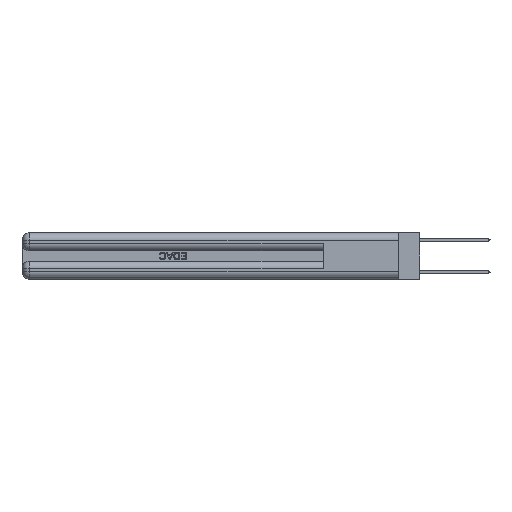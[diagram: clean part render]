
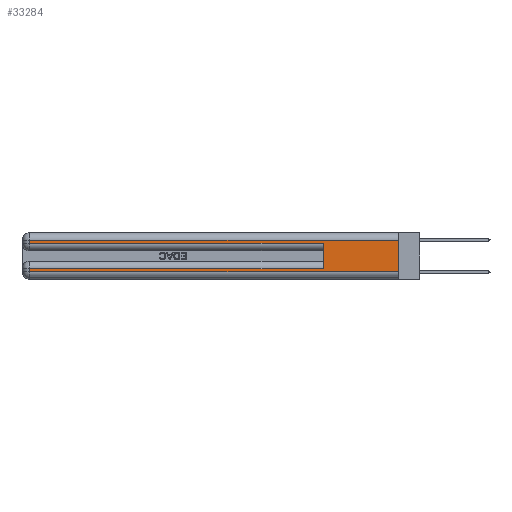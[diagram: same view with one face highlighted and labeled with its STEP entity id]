
A CAD part, left-side view. The second image highlights one B-rep face of the part: STEP entity #33284.
In plain terms, the highlighted planar face has unit normal (-1, 0, 0).
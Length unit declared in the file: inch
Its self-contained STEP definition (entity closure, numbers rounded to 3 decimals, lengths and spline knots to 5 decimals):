
#261 = EDGE_CURVE ( 'NONE', #20659, #24880, #7401, .T. ) ;
#374 = CARTESIAN_POINT ( 'NONE',  ( 0., 0., 0.31 ) ) ;
#693 = CARTESIAN_POINT ( 'NONE',  ( 0., 0.6, 0.285 ) ) ;
#1009 = VECTOR ( 'NONE', #2126, 39.37008 ) ;
#2126 = DIRECTION ( 'NONE',  ( 0., 0., -1. ) ) ;
#2156 = CARTESIAN_POINT ( 'NONE',  ( 0., 2.94, 0.285 ) ) ;
#2361 = DIRECTION ( 'NONE',  ( 0., 0., -1. ) ) ;
#2524 = EDGE_CURVE ( 'NONE', #11188, #22480, #18387, .T. ) ;
#3172 = DIRECTION ( 'NONE',  ( 0., 1., 0. ) ) ;
#3394 = EDGE_CURVE ( 'NONE', #13638, #11188, #4355, .T. ) ;
#3438 = CARTESIAN_POINT ( 'NONE',  ( 0., 0.6, 0.145 ) ) ;
#4263 = EDGE_CURVE ( 'NONE', #24880, #27393, #13263, .T. ) ;
#4355 = LINE ( 'NONE', #27500, #23563 ) ;
#5903 = LINE ( 'NONE', #16945, #30432 ) ;
#7401 = LINE ( 'NONE', #18989, #1009 ) ;
#7465 = CARTESIAN_POINT ( 'NONE',  ( 0., 0., 0.285 ) ) ;
#7902 = CARTESIAN_POINT ( 'NONE',  ( 0., 2.94, 0.085 ) ) ;
#7905 = ORIENTED_EDGE ( 'NONE', *, *, #35413, .F. ) ;
#8218 = ORIENTED_EDGE ( 'NONE', *, *, #4263, .T. ) ;
#10287 = AXIS2_PLACEMENT_3D ( 'NONE', #35179, #10346, #27024 ) ;
#10346 = DIRECTION ( 'NONE',  ( 1., 0., 0. ) ) ;
#10727 = ORIENTED_EDGE ( 'NONE', *, *, #35603, .F. ) ;
#11188 = VERTEX_POINT ( 'NONE', #19655 ) ;
#12116 = VERTEX_POINT ( 'NONE', #20433 ) ;
#12773 = DIRECTION ( 'NONE',  ( 0., 0., -1. ) ) ;
#12913 = VECTOR ( 'NONE', #12773, 39.37008 ) ;
#13059 = PLANE ( 'NONE',  #10287 ) ;
#13263 = LINE ( 'NONE', #21599, #31100 ) ;
#13434 = EDGE_CURVE ( 'NONE', #22480, #21497, #26667, .T. ) ;
#13638 = VERTEX_POINT ( 'NONE', #374 ) ;
#13777 = LINE ( 'NONE', #19567, #30492 ) ;
#14496 = DIRECTION ( 'NONE',  ( 0., 0., 1. ) ) ;
#15276 = CARTESIAN_POINT ( 'NONE',  ( 0., 2.94, 0.06 ) ) ;
#15425 = FACE_OUTER_BOUND ( 'NONE', #23066, .T. ) ;
#15679 = DIRECTION ( 'NONE',  ( 0., 1., 0. ) ) ;
#16455 = ORIENTED_EDGE ( 'NONE', *, *, #261, .T. ) ;
#16945 = CARTESIAN_POINT ( 'NONE',  ( 0., 0., 0.085 ) ) ;
#18325 = DIRECTION ( 'NONE',  ( 0., -1., 0. ) ) ;
#18387 = LINE ( 'NONE', #18565, #12913 ) ;
#18565 = CARTESIAN_POINT ( 'NONE',  ( 0., 2.94, 0.37 ) ) ;
#18989 = CARTESIAN_POINT ( 'NONE',  ( 0., 2.94, 0.37 ) ) ;
#19567 = CARTESIAN_POINT ( 'NONE',  ( 0., 0., 0.37 ) ) ;
#19655 = CARTESIAN_POINT ( 'NONE',  ( 0., 2.94, 0.31 ) ) ;
#20433 = CARTESIAN_POINT ( 'NONE',  ( 0., 0.6, 0.085 ) ) ;
#20659 = VERTEX_POINT ( 'NONE', #7902 ) ;
#21497 = VERTEX_POINT ( 'NONE', #693 ) ;
#21599 = CARTESIAN_POINT ( 'NONE',  ( 0., 0., 0.06 ) ) ;
#21711 = CARTESIAN_POINT ( 'NONE',  ( 0., 0., 0.06 ) ) ;
#22480 = VERTEX_POINT ( 'NONE', #2156 ) ;
#23066 = EDGE_LOOP ( 'NONE', ( #7905, #30994, #31578, #23395, #10727, #25771, #16455, #8218 ) ) ;
#23395 = ORIENTED_EDGE ( 'NONE', *, *, #13434, .T. ) ;
#23563 = VECTOR ( 'NONE', #15679, 39.37008 ) ;
#24298 = VECTOR ( 'NONE', #18325, 39.37008 ) ;
#24880 = VERTEX_POINT ( 'NONE', #15276 ) ;
#25771 = ORIENTED_EDGE ( 'NONE', *, *, #29048, .T. ) ;
#26667 = LINE ( 'NONE', #7465, #24298 ) ;
#27024 = DIRECTION ( 'NONE',  ( 0., 0., -1. ) ) ;
#27222 = DIRECTION ( 'NONE',  ( 0., -1., 0. ) ) ;
#27393 = VERTEX_POINT ( 'NONE', #21711 ) ;
#27500 = CARTESIAN_POINT ( 'NONE',  ( 0., 0., 0.31 ) ) ;
#28162 = VECTOR ( 'NONE', #14496, 39.37008 ) ;
#28273 = LINE ( 'NONE', #3438, #28162 ) ;
#29048 = EDGE_CURVE ( 'NONE', #12116, #20659, #5903, .T. ) ;
#30432 = VECTOR ( 'NONE', #3172, 39.37008 ) ;
#30492 = VECTOR ( 'NONE', #2361, 39.37008 ) ;
#30994 = ORIENTED_EDGE ( 'NONE', *, *, #3394, .T. ) ;
#31100 = VECTOR ( 'NONE', #27222, 39.37008 ) ;
#31578 = ORIENTED_EDGE ( 'NONE', *, *, #2524, .T. ) ;
#33284 = ADVANCED_FACE ( 'NONE', ( #15425 ), #13059, .F. ) ;
#35179 = CARTESIAN_POINT ( 'NONE',  ( 0., 0., 0.37 ) ) ;
#35413 = EDGE_CURVE ( 'NONE', #13638, #27393, #13777, .T. ) ;
#35603 = EDGE_CURVE ( 'NONE', #12116, #21497, #28273, .T. ) ;
